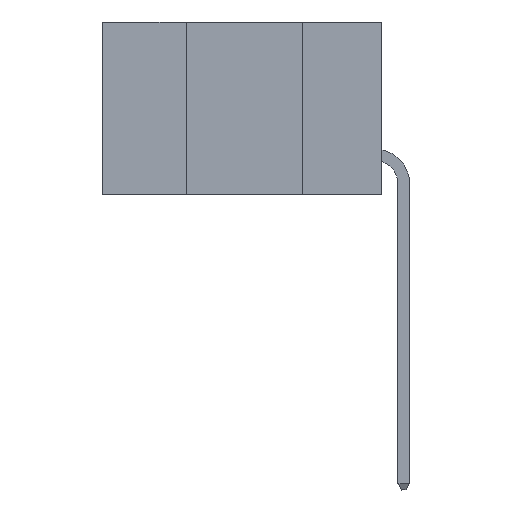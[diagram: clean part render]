
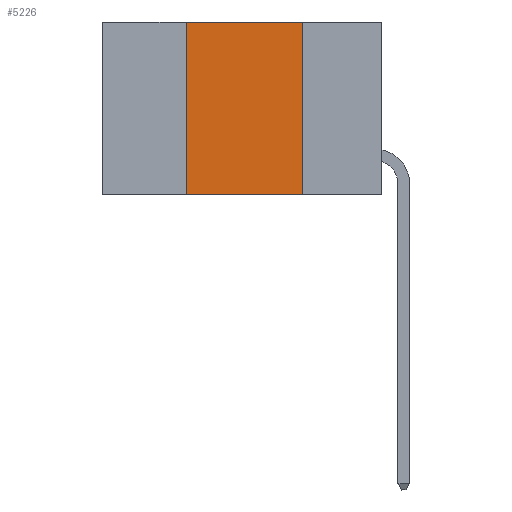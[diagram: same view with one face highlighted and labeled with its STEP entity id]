
A CAD part, left-side view. The second image highlights one B-rep face of the part: STEP entity #5226.
In plain terms, the highlighted planar face has unit normal (-1, 0, 0).
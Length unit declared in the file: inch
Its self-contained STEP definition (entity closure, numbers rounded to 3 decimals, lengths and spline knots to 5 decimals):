
#1665 = VECTOR ( 'NONE', #39175, 39.37008 ) ;
#2613 = CARTESIAN_POINT ( 'NONE',  ( 0., 0.6, 0. ) ) ;
#2935 = LINE ( 'NONE', #2613, #27188 ) ;
#4438 = CARTESIAN_POINT ( 'NONE',  ( 0., 0.17, -0.37 ) ) ;
#5226 = ADVANCED_FACE ( 'NONE', ( #11331 ), #9751, .F. ) ;
#5953 = CARTESIAN_POINT ( 'NONE',  ( 0., 0.42, 0. ) ) ;
#7649 = ORIENTED_EDGE ( 'NONE', *, *, #19774, .F. ) ;
#7827 = VERTEX_POINT ( 'NONE', #39187 ) ;
#8923 = EDGE_CURVE ( 'NONE', #7827, #12033, #28861, .T. ) ;
#9173 = CARTESIAN_POINT ( 'NONE',  ( 0., 0.6, -0.37 ) ) ;
#9751 = PLANE ( 'NONE',  #29737 ) ;
#10073 = CARTESIAN_POINT ( 'NONE',  ( 0., 0.6, 0. ) ) ;
#11331 = FACE_OUTER_BOUND ( 'NONE', #15481, .T. ) ;
#12033 = VERTEX_POINT ( 'NONE', #4438 ) ;
#13519 = DIRECTION ( 'NONE',  ( 0., 0., -1. ) ) ;
#15167 = DIRECTION ( 'NONE',  ( 0., -1., 0. ) ) ;
#15481 = EDGE_LOOP ( 'NONE', ( #23491, #19312, #7649, #41540 ) ) ;
#19312 = ORIENTED_EDGE ( 'NONE', *, *, #38719, .F. ) ;
#19774 = EDGE_CURVE ( 'NONE', #7827, #28205, #30991, .T. ) ;
#23491 = ORIENTED_EDGE ( 'NONE', *, *, #48843, .F. ) ;
#24795 = LINE ( 'NONE', #44746, #43830 ) ;
#25112 = DIRECTION ( 'NONE',  ( 0., 0., 1. ) ) ;
#25140 = DIRECTION ( 'NONE',  ( 0., 0., -1. ) ) ;
#27188 = VECTOR ( 'NONE', #15167, 39.37008 ) ;
#28205 = VERTEX_POINT ( 'NONE', #28886 ) ;
#28861 = LINE ( 'NONE', #9173, #1665 ) ;
#28886 = CARTESIAN_POINT ( 'NONE',  ( 0., 0.42, 0. ) ) ;
#29737 = AXIS2_PLACEMENT_3D ( 'NONE', #10073, #43761, #13519 ) ;
#30991 = LINE ( 'NONE', #5953, #41726 ) ;
#31926 = VERTEX_POINT ( 'NONE', #37586 ) ;
#37586 = CARTESIAN_POINT ( 'NONE',  ( 0., 0.17, 0. ) ) ;
#38719 = EDGE_CURVE ( 'NONE', #28205, #31926, #2935, .T. ) ;
#39175 = DIRECTION ( 'NONE',  ( 0., -1., 0. ) ) ;
#39187 = CARTESIAN_POINT ( 'NONE',  ( 0., 0.42, -0.37 ) ) ;
#41540 = ORIENTED_EDGE ( 'NONE', *, *, #8923, .T. ) ;
#41726 = VECTOR ( 'NONE', #25112, 39.37008 ) ;
#43761 = DIRECTION ( 'NONE',  ( 1., 0., 0. ) ) ;
#43830 = VECTOR ( 'NONE', #25140, 39.37008 ) ;
#44746 = CARTESIAN_POINT ( 'NONE',  ( 0., 0.17, 0. ) ) ;
#48843 = EDGE_CURVE ( 'NONE', #31926, #12033, #24795, .T. ) ;
